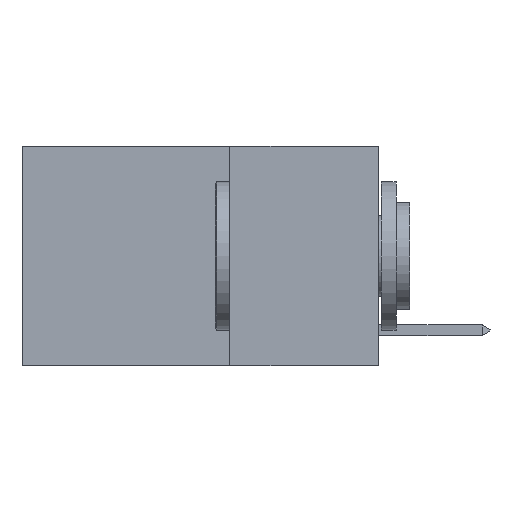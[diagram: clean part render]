
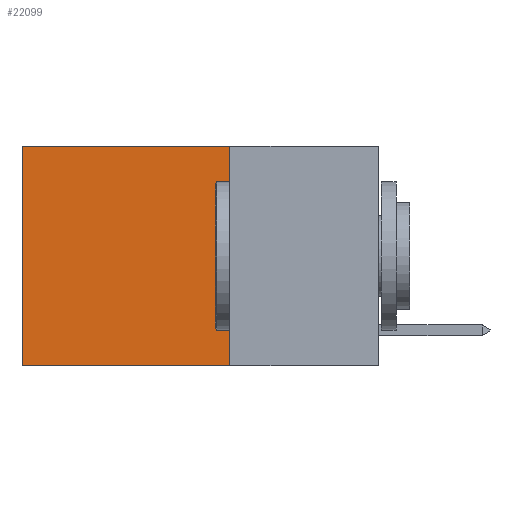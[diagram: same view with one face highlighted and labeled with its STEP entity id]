
A CAD part, left-side view. The second image highlights one B-rep face of the part: STEP entity #22099.
In plain terms, the highlighted planar face has unit normal (-1, 0, 0).
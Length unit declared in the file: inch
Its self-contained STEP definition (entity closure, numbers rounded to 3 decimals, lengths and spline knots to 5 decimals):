
#50 = DIRECTION ( 'NONE',  ( 0., 0., -1. ) ) ;
#191 = DIRECTION ( 'NONE',  ( 0., 1., 0. ) ) ;
#505 = DIRECTION ( 'NONE',  ( 0., 0., -1. ) ) ;
#1192 = CARTESIAN_POINT ( 'NONE',  ( 0.2625, 0.25, -0.37 ) ) ;
#2487 = LINE ( 'NONE', #10641, #8336 ) ;
#3033 = EDGE_LOOP ( 'NONE', ( #24226, #17275, #9492, #4246 ) ) ;
#3432 = VERTEX_POINT ( 'NONE', #1192 ) ;
#4246 = ORIENTED_EDGE ( 'NONE', *, *, #7281, .T. ) ;
#5012 = EDGE_CURVE ( 'NONE', #20430, #23839, #2487, .T. ) ;
#7281 = EDGE_CURVE ( 'NONE', #10723, #20430, #18446, .T. ) ;
#7849 = CARTESIAN_POINT ( 'NONE',  ( 0.2625, 0.6, 0. ) ) ;
#8013 = LINE ( 'NONE', #16129, #25719 ) ;
#8336 = VECTOR ( 'NONE', #505, 39.37008 ) ;
#8461 = CARTESIAN_POINT ( 'NONE',  ( 0.2625, 0.25, 0. ) ) ;
#9010 = VECTOR ( 'NONE', #191, 39.37008 ) ;
#9492 = ORIENTED_EDGE ( 'NONE', *, *, #12341, .F. ) ;
#10641 = CARTESIAN_POINT ( 'NONE',  ( 0.2625, 0.6, 0. ) ) ;
#10723 = VERTEX_POINT ( 'NONE', #21104 ) ;
#12341 = EDGE_CURVE ( 'NONE', #10723, #3432, #26263, .T. ) ;
#16129 = CARTESIAN_POINT ( 'NONE',  ( 0.2625, 0.25, -0.37 ) ) ;
#16193 = CARTESIAN_POINT ( 'NONE',  ( 0.2625, 0.25, 0. ) ) ;
#16283 = EDGE_CURVE ( 'NONE', #3432, #23839, #8013, .T. ) ;
#16584 = DIRECTION ( 'NONE',  ( 1., 0., 0. ) ) ;
#17275 = ORIENTED_EDGE ( 'NONE', *, *, #16283, .F. ) ;
#18178 = PLANE ( 'NONE',  #20228 ) ;
#18446 = LINE ( 'NONE', #24549, #9010 ) ;
#18572 = FACE_OUTER_BOUND ( 'NONE', #3033, .T. ) ;
#18855 = VECTOR ( 'NONE', #50, 39.37008 ) ;
#20228 = AXIS2_PLACEMENT_3D ( 'NONE', #8461, #16584, #26136 ) ;
#20430 = VERTEX_POINT ( 'NONE', #7849 ) ;
#21104 = CARTESIAN_POINT ( 'NONE',  ( 0.2625, 0.25, 0. ) ) ;
#22099 = ADVANCED_FACE ( 'NONE', ( #18572 ), #18178, .F. ) ;
#22256 = CARTESIAN_POINT ( 'NONE',  ( 0.2625, 0.6, -0.37 ) ) ;
#23839 = VERTEX_POINT ( 'NONE', #22256 ) ;
#24209 = DIRECTION ( 'NONE',  ( 0., 1., 0. ) ) ;
#24226 = ORIENTED_EDGE ( 'NONE', *, *, #5012, .T. ) ;
#24549 = CARTESIAN_POINT ( 'NONE',  ( 0.2625, 0.25, 0. ) ) ;
#25719 = VECTOR ( 'NONE', #24209, 39.37008 ) ;
#26136 = DIRECTION ( 'NONE',  ( 0., 0., -1. ) ) ;
#26263 = LINE ( 'NONE', #16193, #18855 ) ;
